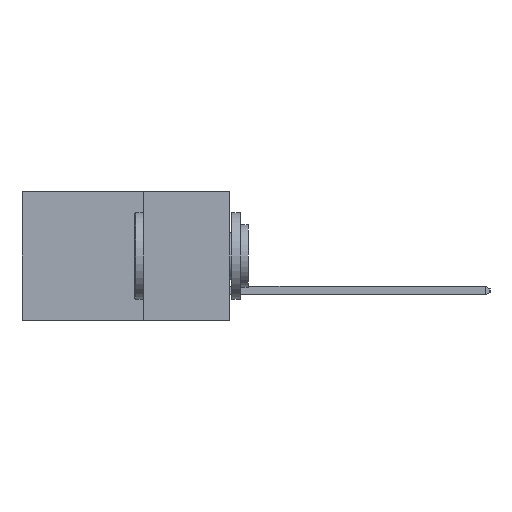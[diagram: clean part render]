
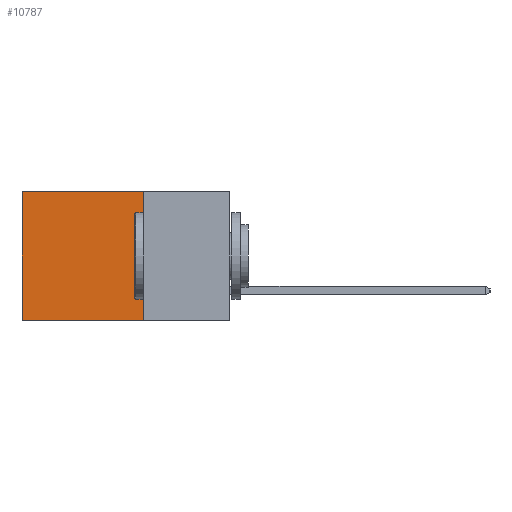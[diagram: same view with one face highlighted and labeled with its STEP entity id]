
A CAD part, left-side view. The second image highlights one B-rep face of the part: STEP entity #10787.
In plain terms, the highlighted planar face has unit normal (-1, 0, 0).
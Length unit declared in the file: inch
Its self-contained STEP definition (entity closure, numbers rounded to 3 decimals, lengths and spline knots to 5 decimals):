
#148 = DIRECTION ( 'NONE',  ( 0., 0., -1. ) ) ;
#257 = CARTESIAN_POINT ( 'NONE',  ( 0.298, 0.6, -0.37 ) ) ;
#456 = CARTESIAN_POINT ( 'NONE',  ( 0.298, 0.25, -0.37 ) ) ;
#781 = LINE ( 'NONE', #8517, #3078 ) ;
#1849 = VERTEX_POINT ( 'NONE', #257 ) ;
#2084 = PLANE ( 'NONE',  #2638 ) ;
#2311 = DIRECTION ( 'NONE',  ( 0., 0., -1. ) ) ;
#2638 = AXIS2_PLACEMENT_3D ( 'NONE', #10747, #5801, #148 ) ;
#2642 = DIRECTION ( 'NONE',  ( 0., 1., 0. ) ) ;
#2737 = VECTOR ( 'NONE', #4340, 39.37008 ) ;
#2872 = EDGE_CURVE ( 'NONE', #3552, #3820, #4327, .T. ) ;
#2997 = EDGE_LOOP ( 'NONE', ( #3962, #3992, #4013, #4040 ) ) ;
#3078 = VECTOR ( 'NONE', #2311, 39.37008 ) ;
#3552 = VERTEX_POINT ( 'NONE', #3584 ) ;
#3584 = CARTESIAN_POINT ( 'NONE',  ( 0.298, 0.25, 0. ) ) ;
#3820 = VERTEX_POINT ( 'NONE', #4683 ) ;
#3962 = ORIENTED_EDGE ( 'NONE', *, *, #10454, .T. ) ;
#3992 = ORIENTED_EDGE ( 'NONE', *, *, #9910, .F. ) ;
#4013 = ORIENTED_EDGE ( 'NONE', *, *, #9115, .F. ) ;
#4040 = ORIENTED_EDGE ( 'NONE', *, *, #2872, .T. ) ;
#4327 = LINE ( 'NONE', #8156, #8420 ) ;
#4340 = DIRECTION ( 'NONE',  ( 0., 0., -1. ) ) ;
#4683 = CARTESIAN_POINT ( 'NONE',  ( 0.298, 0.6, 0. ) ) ;
#5372 = CARTESIAN_POINT ( 'NONE',  ( 0.298, 0.25, -0.37 ) ) ;
#5757 = FACE_OUTER_BOUND ( 'NONE', #2997, .T. ) ;
#5801 = DIRECTION ( 'NONE',  ( 1., 0., 0. ) ) ;
#6927 = VECTOR ( 'NONE', #2642, 39.37008 ) ;
#6997 = DIRECTION ( 'NONE',  ( 0., 1., 0. ) ) ;
#7077 = CARTESIAN_POINT ( 'NONE',  ( 0.298, 0.6, 0. ) ) ;
#7188 = LINE ( 'NONE', #5372, #6927 ) ;
#7496 = VERTEX_POINT ( 'NONE', #456 ) ;
#7585 = LINE ( 'NONE', #7077, #2737 ) ;
#8156 = CARTESIAN_POINT ( 'NONE',  ( 0.298, 0.25, 0. ) ) ;
#8420 = VECTOR ( 'NONE', #6997, 39.37008 ) ;
#8517 = CARTESIAN_POINT ( 'NONE',  ( 0.298, 0.25, 0. ) ) ;
#9115 = EDGE_CURVE ( 'NONE', #3552, #7496, #781, .T. ) ;
#9910 = EDGE_CURVE ( 'NONE', #7496, #1849, #7188, .T. ) ;
#10454 = EDGE_CURVE ( 'NONE', #3820, #1849, #7585, .T. ) ;
#10747 = CARTESIAN_POINT ( 'NONE',  ( 0.298, 0.25, 0. ) ) ;
#10787 = ADVANCED_FACE ( 'NONE', ( #5757 ), #2084, .F. ) ;
